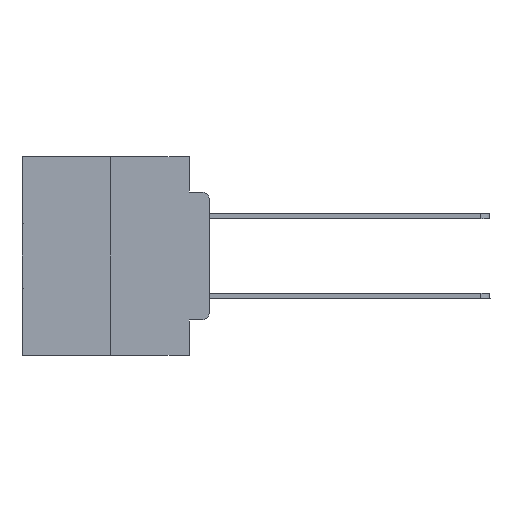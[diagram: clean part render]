
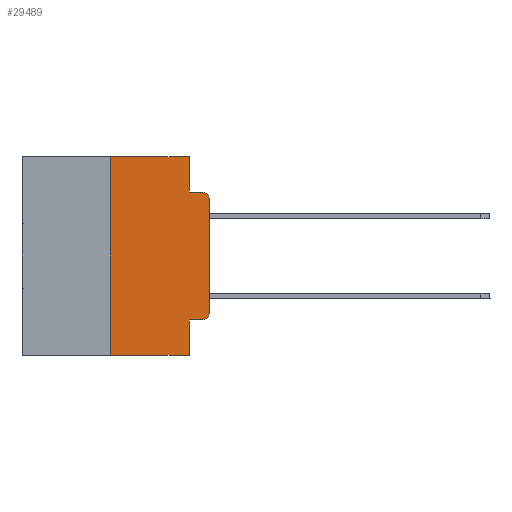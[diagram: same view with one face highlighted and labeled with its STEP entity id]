
A CAD part, left-side view. The second image highlights one B-rep face of the part: STEP entity #29489.
In plain terms, the highlighted planar face has unit normal (-1, 0, 0).
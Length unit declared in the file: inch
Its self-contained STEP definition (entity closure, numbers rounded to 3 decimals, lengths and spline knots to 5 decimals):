
#961 = VECTOR ( 'NONE', #3962, 39.37008 ) ;
#1389 = ORIENTED_EDGE ( 'NONE', *, *, #11491, .F. ) ;
#1499 = CARTESIAN_POINT ( 'NONE',  ( 0., 0.051, -0.4115 ) ) ;
#2078 = EDGE_CURVE ( 'NONE', #15592, #19110, #29515, .T. ) ;
#2278 = LINE ( 'NONE', #6708, #27452 ) ;
#2820 = DIRECTION ( 'NONE',  ( 0., 0., 1. ) ) ;
#2923 = EDGE_CURVE ( 'NONE', #16945, #29674, #8557, .T. ) ;
#3514 = ORIENTED_EDGE ( 'NONE', *, *, #7848, .T. ) ;
#3661 = CARTESIAN_POINT ( 'NONE',  ( 0., 0., -0.1085 ) ) ;
#3846 = CARTESIAN_POINT ( 'NONE',  ( 0., 0.051, -0.0885 ) ) ;
#3962 = DIRECTION ( 'NONE',  ( 0., -1., 0. ) ) ;
#4040 = DIRECTION ( 'NONE',  ( 0., 0., -1. ) ) ;
#4263 = ORIENTED_EDGE ( 'NONE', *, *, #10262, .F. ) ;
#4710 = DIRECTION ( 'NONE',  ( -1., 0., 0. ) ) ;
#5064 = VERTEX_POINT ( 'NONE', #18934 ) ;
#5139 = DIRECTION ( 'NONE',  ( 0., 0., -1. ) ) ;
#5153 = ORIENTED_EDGE ( 'NONE', *, *, #28510, .T. ) ;
#5739 = EDGE_CURVE ( 'NONE', #27539, #9624, #25047, .T. ) ;
#5883 = LINE ( 'NONE', #20515, #20691 ) ;
#6012 = ORIENTED_EDGE ( 'NONE', *, *, #24677, .T. ) ;
#6219 = DIRECTION ( 'NONE',  ( 0., 0., -1. ) ) ;
#6708 = CARTESIAN_POINT ( 'NONE',  ( 0., 0.473, -0.5 ) ) ;
#7848 = EDGE_CURVE ( 'NONE', #5064, #13901, #17515, .T. ) ;
#8124 = ORIENTED_EDGE ( 'NONE', *, *, #17117, .T. ) ;
#8557 = CIRCLE ( 'NONE', #11678, 0.02 ) ;
#9004 = DIRECTION ( 'NONE',  ( 0., 0., 1. ) ) ;
#9473 = DIRECTION ( 'NONE',  ( 0., -1., 0. ) ) ;
#9624 = VERTEX_POINT ( 'NONE', #3846 ) ;
#10262 = EDGE_CURVE ( 'NONE', #19110, #27539, #28854, .T. ) ;
#10459 = AXIS2_PLACEMENT_3D ( 'NONE', #25383, #10792, #6219 ) ;
#10721 = CARTESIAN_POINT ( 'NONE',  ( 0., 0., -0.3915 ) ) ;
#10792 = DIRECTION ( 'NONE',  ( 1., 0., 0. ) ) ;
#10872 = LINE ( 'NONE', #28373, #961 ) ;
#11491 = EDGE_CURVE ( 'NONE', #9624, #29674, #10872, .T. ) ;
#11517 = DIRECTION ( 'NONE',  ( 0., -1., 0. ) ) ;
#11569 = LINE ( 'NONE', #28592, #28726 ) ;
#11599 = CARTESIAN_POINT ( 'NONE',  ( 0., 0.473, 0. ) ) ;
#11678 = AXIS2_PLACEMENT_3D ( 'NONE', #19998, #15099, #5139 ) ;
#11691 = VERTEX_POINT ( 'NONE', #29780 ) ;
#12596 = ORIENTED_EDGE ( 'NONE', *, *, #2078, .F. ) ;
#12992 = CARTESIAN_POINT ( 'NONE',  ( 0., 0.051, 0. ) ) ;
#13013 = ORIENTED_EDGE ( 'NONE', *, *, #2923, .T. ) ;
#13901 = VERTEX_POINT ( 'NONE', #10721 ) ;
#15099 = DIRECTION ( 'NONE',  ( -1., 0., 0. ) ) ;
#15369 = EDGE_LOOP ( 'NONE', ( #8124, #13013, #1389, #20234, #4263, #12596, #5153, #27707, #6012, #3514 ) ) ;
#15592 = VERTEX_POINT ( 'NONE', #24697 ) ;
#15721 = VECTOR ( 'NONE', #11517, 39.37008 ) ;
#15811 = EDGE_CURVE ( 'NONE', #25070, #11691, #5883, .T. ) ;
#16945 = VERTEX_POINT ( 'NONE', #3661 ) ;
#17117 = EDGE_CURVE ( 'NONE', #13901, #16945, #11569, .T. ) ;
#17515 = CIRCLE ( 'NONE', #26874, 0.02 ) ;
#17887 = CARTESIAN_POINT ( 'NONE',  ( 0., 0.051, 0. ) ) ;
#17917 = CARTESIAN_POINT ( 'NONE',  ( 0., 0.25, 0. ) ) ;
#18934 = CARTESIAN_POINT ( 'NONE',  ( 0., 0.02, -0.4115 ) ) ;
#19110 = VERTEX_POINT ( 'NONE', #17917 ) ;
#19446 = DIRECTION ( 'NONE',  ( 0., 0., -1. ) ) ;
#19998 = CARTESIAN_POINT ( 'NONE',  ( 0., 0.02, -0.1085 ) ) ;
#20234 = ORIENTED_EDGE ( 'NONE', *, *, #5739, .F. ) ;
#20515 = CARTESIAN_POINT ( 'NONE',  ( 0., 0.051, 0. ) ) ;
#20691 = VECTOR ( 'NONE', #4040, 39.37008 ) ;
#20758 = PLANE ( 'NONE',  #10459 ) ;
#20959 = CARTESIAN_POINT ( 'NONE',  ( 0., 0.02, -0.0885 ) ) ;
#22263 = CARTESIAN_POINT ( 'NONE',  ( 0., 0.25, 0. ) ) ;
#23558 = FACE_OUTER_BOUND ( 'NONE', #15369, .T. ) ;
#24677 = EDGE_CURVE ( 'NONE', #25070, #5064, #31078, .T. ) ;
#24697 = CARTESIAN_POINT ( 'NONE',  ( 0., 0.25, -0.5 ) ) ;
#25047 = LINE ( 'NONE', #12992, #29584 ) ;
#25070 = VERTEX_POINT ( 'NONE', #29968 ) ;
#25279 = DIRECTION ( 'NONE',  ( 0., 0., -1. ) ) ;
#25383 = CARTESIAN_POINT ( 'NONE',  ( 0., 0.473, 0. ) ) ;
#25743 = VECTOR ( 'NONE', #31152, 39.37008 ) ;
#26874 = AXIS2_PLACEMENT_3D ( 'NONE', #31601, #4710, #19446 ) ;
#27203 = VECTOR ( 'NONE', #2820, 39.37008 ) ;
#27452 = VECTOR ( 'NONE', #9473, 39.37008 ) ;
#27539 = VERTEX_POINT ( 'NONE', #17887 ) ;
#27707 = ORIENTED_EDGE ( 'NONE', *, *, #15811, .F. ) ;
#28373 = CARTESIAN_POINT ( 'NONE',  ( 0., 0.051, -0.0885 ) ) ;
#28510 = EDGE_CURVE ( 'NONE', #15592, #11691, #2278, .T. ) ;
#28592 = CARTESIAN_POINT ( 'NONE',  ( 0., 0., 0. ) ) ;
#28726 = VECTOR ( 'NONE', #9004, 39.37008 ) ;
#28854 = LINE ( 'NONE', #11599, #25743 ) ;
#29489 = ADVANCED_FACE ( 'NONE', ( #23558 ), #20758, .F. ) ;
#29515 = LINE ( 'NONE', #22263, #27203 ) ;
#29584 = VECTOR ( 'NONE', #25279, 39.37008 ) ;
#29674 = VERTEX_POINT ( 'NONE', #20959 ) ;
#29780 = CARTESIAN_POINT ( 'NONE',  ( 0., 0.051, -0.5 ) ) ;
#29968 = CARTESIAN_POINT ( 'NONE',  ( 0., 0.051, -0.4115 ) ) ;
#31078 = LINE ( 'NONE', #1499, #15721 ) ;
#31152 = DIRECTION ( 'NONE',  ( 0., -1., 0. ) ) ;
#31601 = CARTESIAN_POINT ( 'NONE',  ( 0., 0.02, -0.3915 ) ) ;
